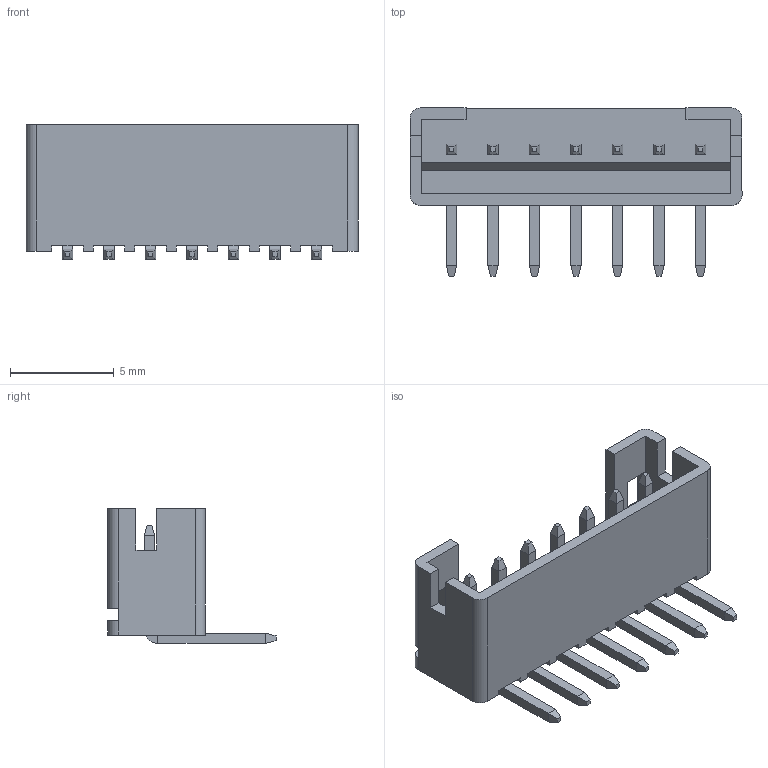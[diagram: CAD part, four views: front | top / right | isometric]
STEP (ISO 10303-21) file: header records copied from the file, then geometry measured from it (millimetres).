
FILE_DESCRIPTION (( 'STEP AP203' ), '1' );
FILE_NAME ('140-507-415-100.STEP', '2020-09-25T11:00:01', ( '' ), ( '' ), 'SwSTEP 2.0', 'SolidWorks 2020', '' );
FILE_SCHEMA (( 'CONFIG_CONTROL_DESIGN' ));
Length unit declared in the file: millimetre
Products named in the file (3): RA LI Contact_Str; 140-507-415-100; RA LI Housing_507
Assembly tree (8 placements, depth 2):
  140-507-415-100
    RA LI Housing_507
    RA LI Contact_Str  x7
Bounding box: 16 x 8.1 x 6.5 mm (x, y, z)
Volume: 180.5 mm3; surface area: 682.1 mm2
Topology: 8 solids, 8 shells, 250 faces, 592 edges, 356 vertices
Faces by surface type: plane 230, cylinder 20
Entity records: 4221 total; most frequent: CARTESIAN_POINT 669, ORIENTED_EDGE 656, DIRECTION 602, EDGE_CURVE 328, LINE 312, VECTOR 312, VERTEX_POINT 212, AXIS2_PLACEMENT_3D 145
